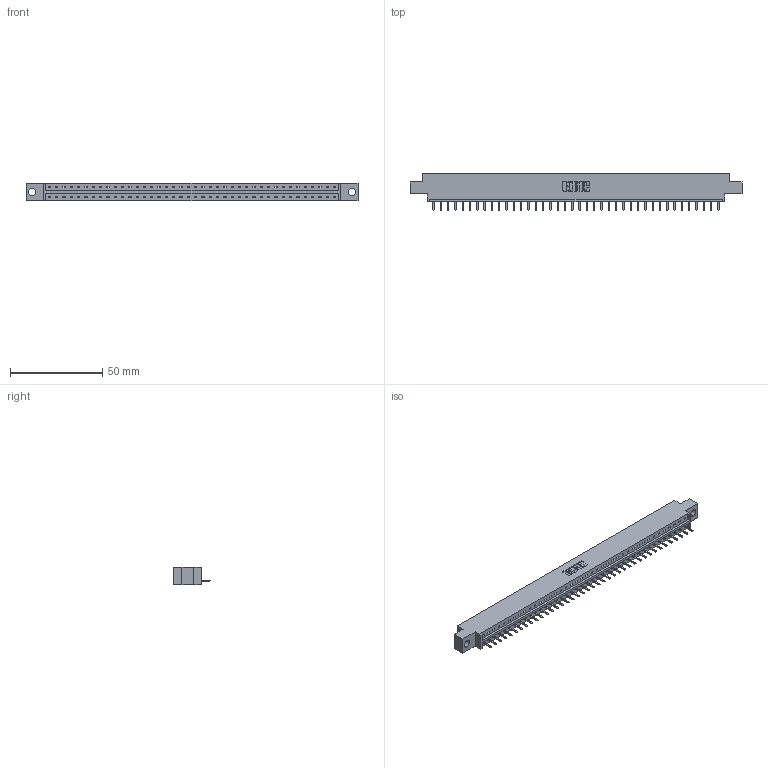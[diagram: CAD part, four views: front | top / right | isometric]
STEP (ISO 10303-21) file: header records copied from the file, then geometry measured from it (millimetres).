
FILE_DESCRIPTION (( 'STEP AP203' ), '1' );
FILE_NAME ('333-040-520-604.STEP', '2018-08-03T13:33:48', ( '' ), ( '' ), 'SwSTEP 2.0', 'SolidWorks 2016', '' );
FILE_SCHEMA (( 'CONFIG_CONTROL_DESIGN' ));
Length unit declared in the file: inch
Products named in the file (3): 345-292-001_345-293-120; 333-040-520-604; 333 Part_Offset - .156 Dia - TH
Assembly tree (41 placements, depth 2):
  333-040-520-604
    333 Part_Offset - .156 Dia - TH
    345-292-001_345-293-120  x40
Bounding box: 180.04 x 20.02 x 9.4 mm (x, y, z)
Volume: 17668.7 mm3; surface area: 18693.9 mm2
Topology: 41 solids, 41 shells, 2598 faces, 7683 edges, 5014 vertices
Faces by surface type: plane 1834, cylinder 764
Entity records: 24961 total; most frequent: CARTESIAN_POINT 4326, ORIENTED_EDGE 4290, DIRECTION 3641, EDGE_CURVE 2145, VECTOR 2013, LINE 2013, VERTEX_POINT 1426, AXIS2_PLACEMENT_3D 814
